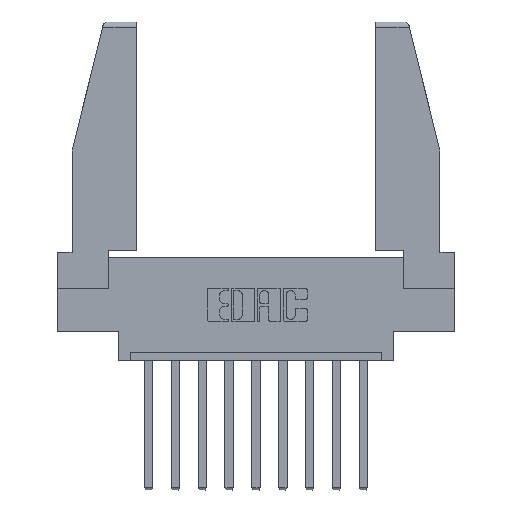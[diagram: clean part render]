
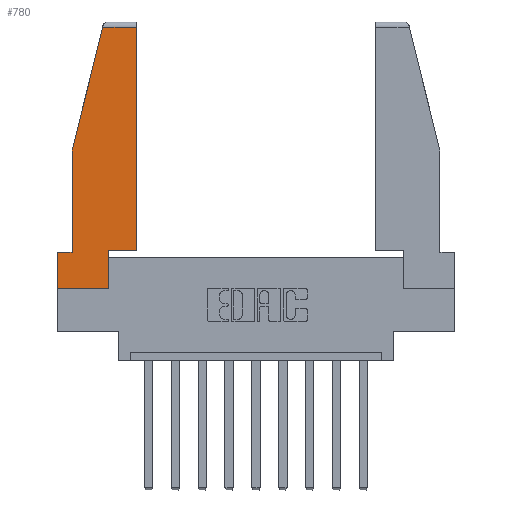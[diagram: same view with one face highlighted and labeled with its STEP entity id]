
A CAD part, top view. The second image highlights one B-rep face of the part: STEP entity #780.
In plain terms, the highlighted planar face has unit normal (0, 0, 1).
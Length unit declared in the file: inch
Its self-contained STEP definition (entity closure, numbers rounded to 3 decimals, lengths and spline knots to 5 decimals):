
#53 = EDGE_CURVE ( 'NONE', #2171, #7022, #1017, .T. ) ;
#125 = VECTOR ( 'NONE', #1577, 39.37008 ) ;
#165 = CARTESIAN_POINT ( 'NONE',  ( 0.461, 0.223, 0. ) ) ;
#647 = DIRECTION ( 'NONE',  ( 0., 0., 1. ) ) ;
#770 = EDGE_CURVE ( 'NONE', #9913, #11845, #3066, .T. ) ;
#780 = ADVANCED_FACE ( 'NONE', ( #11645 ), #10798, .T. ) ;
#837 = EDGE_LOOP ( 'NONE', ( #1333, #6442, #12371, #971, #10793, #3717, #6523, #12695, #11663 ) ) ;
#971 = ORIENTED_EDGE ( 'NONE', *, *, #7253, .T. ) ;
#1017 = LINE ( 'NONE', #4268, #11674 ) ;
#1269 = VERTEX_POINT ( 'NONE', #165 ) ;
#1333 = ORIENTED_EDGE ( 'NONE', *, *, #5027, .T. ) ;
#1577 = DIRECTION ( 'NONE',  ( -1., 0., 0. ) ) ;
#2171 = VERTEX_POINT ( 'NONE', #9368 ) ;
#2265 = AXIS2_PLACEMENT_3D ( 'NONE', #10927, #647, #11886 ) ;
#2314 = CARTESIAN_POINT ( 'NONE',  ( 0.461, 0.223, 0. ) ) ;
#2847 = LINE ( 'NONE', #7762, #125 ) ;
#2974 = DIRECTION ( 'NONE',  ( 0., -1., 0. ) ) ;
#3066 = LINE ( 'NONE', #9898, #9215 ) ;
#3179 = EDGE_CURVE ( 'NONE', #6715, #5666, #2847, .T. ) ;
#3212 = CARTESIAN_POINT ( 'NONE',  ( 0.086, 0.21, 0. ) ) ;
#3517 = EDGE_CURVE ( 'NONE', #12250, #2171, #8299, .T. ) ;
#3717 = ORIENTED_EDGE ( 'NONE', *, *, #8408, .T. ) ;
#3967 = VECTOR ( 'NONE', #5388, 39.37008 ) ;
#4268 = CARTESIAN_POINT ( 'NONE',  ( 0.297, 0., 0. ) ) ;
#4339 = DIRECTION ( 'NONE',  ( 1., 0., 0. ) ) ;
#4615 = VECTOR ( 'NONE', #4339, 39.37008 ) ;
#4756 = CARTESIAN_POINT ( 'NONE',  ( 0.2636, 1.52, 0. ) ) ;
#5027 = EDGE_CURVE ( 'NONE', #1269, #8622, #13286, .T. ) ;
#5263 = LINE ( 'NONE', #7507, #3967 ) ;
#5386 = CARTESIAN_POINT ( 'NONE',  ( 0., 1.52, 0. ) ) ;
#5388 = DIRECTION ( 'NONE',  ( 0., -1., 0. ) ) ;
#5437 = CARTESIAN_POINT ( 'NONE',  ( 0.297, 0.223, 0. ) ) ;
#5634 = CARTESIAN_POINT ( 'NONE',  ( 0., 0.21, 0. ) ) ;
#5666 = VERTEX_POINT ( 'NONE', #5634 ) ;
#5738 = DIRECTION ( 'NONE',  ( -0.239, -0.971, 0. ) ) ;
#6040 = CARTESIAN_POINT ( 'NONE',  ( 0.086, 0.8, 0. ) ) ;
#6102 = CARTESIAN_POINT ( 'NONE',  ( 0., 0., 0. ) ) ;
#6239 = DIRECTION ( 'NONE',  ( 0., 1., 0. ) ) ;
#6341 = CARTESIAN_POINT ( 'NONE',  ( 0.086, 0.8, 0. ) ) ;
#6442 = ORIENTED_EDGE ( 'NONE', *, *, #13139, .T. ) ;
#6523 = ORIENTED_EDGE ( 'NONE', *, *, #3517, .T. ) ;
#6715 = VERTEX_POINT ( 'NONE', #3212 ) ;
#6764 = VECTOR ( 'NONE', #12499, 39.37008 ) ;
#6880 = CARTESIAN_POINT ( 'NONE',  ( 0.297, 0.223, 0. ) ) ;
#7022 = VERTEX_POINT ( 'NONE', #6880 ) ;
#7253 = EDGE_CURVE ( 'NONE', #11845, #6715, #10949, .T. ) ;
#7507 = CARTESIAN_POINT ( 'NONE',  ( 0., 0.21, 0. ) ) ;
#7762 = CARTESIAN_POINT ( 'NONE',  ( 0., 0.21, 0. ) ) ;
#8128 = VECTOR ( 'NONE', #6239, 39.37008 ) ;
#8144 = VECTOR ( 'NONE', #12316, 39.37008 ) ;
#8216 = VECTOR ( 'NONE', #2974, 39.37008 ) ;
#8299 = LINE ( 'NONE', #10370, #8144 ) ;
#8387 = EDGE_CURVE ( 'NONE', #7022, #1269, #10112, .T. ) ;
#8392 = DIRECTION ( 'NONE',  ( 0., 1., 0. ) ) ;
#8408 = EDGE_CURVE ( 'NONE', #5666, #12250, #5263, .T. ) ;
#8622 = VERTEX_POINT ( 'NONE', #12588 ) ;
#9215 = VECTOR ( 'NONE', #5738, 39.37008 ) ;
#9368 = CARTESIAN_POINT ( 'NONE',  ( 0.297, 0., 0. ) ) ;
#9898 = CARTESIAN_POINT ( 'NONE',  ( 0.271, 1.55, 0. ) ) ;
#9913 = VERTEX_POINT ( 'NONE', #4756 ) ;
#10112 = LINE ( 'NONE', #5437, #4615 ) ;
#10370 = CARTESIAN_POINT ( 'NONE',  ( 0., 0., 0. ) ) ;
#10793 = ORIENTED_EDGE ( 'NONE', *, *, #3179, .T. ) ;
#10798 = PLANE ( 'NONE',  #2265 ) ;
#10927 = CARTESIAN_POINT ( 'NONE',  ( 0., 0., 0. ) ) ;
#10949 = LINE ( 'NONE', #6040, #8216 ) ;
#11283 = LINE ( 'NONE', #5386, #6764 ) ;
#11645 = FACE_OUTER_BOUND ( 'NONE', #837, .T. ) ;
#11663 = ORIENTED_EDGE ( 'NONE', *, *, #8387, .T. ) ;
#11674 = VECTOR ( 'NONE', #8392, 39.37008 ) ;
#11845 = VERTEX_POINT ( 'NONE', #6341 ) ;
#11886 = DIRECTION ( 'NONE',  ( 1., 0., 0. ) ) ;
#12250 = VERTEX_POINT ( 'NONE', #6102 ) ;
#12316 = DIRECTION ( 'NONE',  ( 1., 0., 0. ) ) ;
#12371 = ORIENTED_EDGE ( 'NONE', *, *, #770, .T. ) ;
#12499 = DIRECTION ( 'NONE',  ( -1., 0., 0. ) ) ;
#12588 = CARTESIAN_POINT ( 'NONE',  ( 0.461, 1.52, 0. ) ) ;
#12695 = ORIENTED_EDGE ( 'NONE', *, *, #53, .T. ) ;
#13139 = EDGE_CURVE ( 'NONE', #8622, #9913, #11283, .T. ) ;
#13286 = LINE ( 'NONE', #2314, #8128 ) ;
